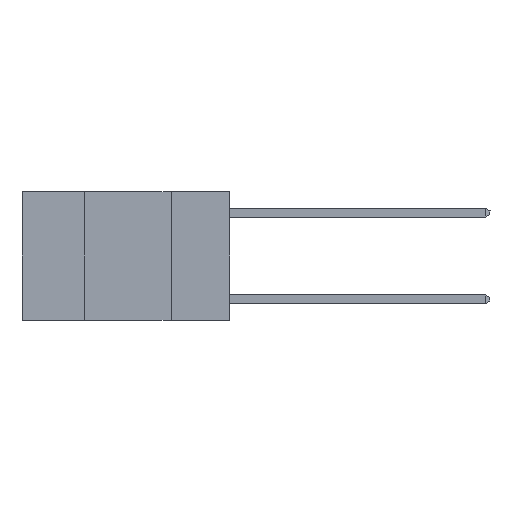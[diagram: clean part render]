
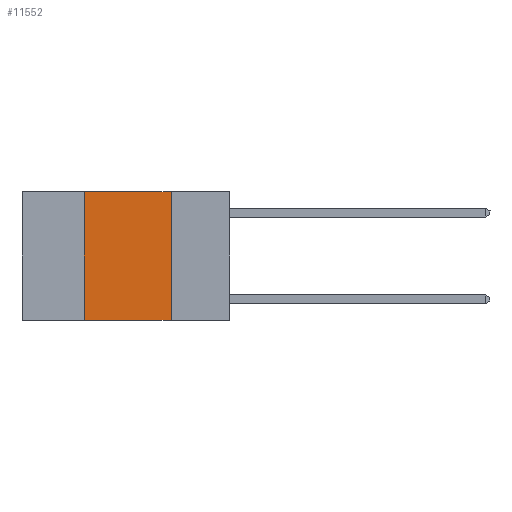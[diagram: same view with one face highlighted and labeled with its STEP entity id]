
A CAD part, left-side view. The second image highlights one B-rep face of the part: STEP entity #11552.
In plain terms, the highlighted planar face has unit normal (-1, 0, 0).
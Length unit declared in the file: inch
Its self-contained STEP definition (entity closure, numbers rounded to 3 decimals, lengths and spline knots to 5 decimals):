
#292 = LINE ( 'NONE', #2393, #14586 ) ;
#581 = CARTESIAN_POINT ( 'NONE',  ( 0., 0.17, -0.37 ) ) ;
#664 = EDGE_CURVE ( 'NONE', #5744, #1374, #12304, .T. ) ;
#1374 = VERTEX_POINT ( 'NONE', #581 ) ;
#2301 = VECTOR ( 'NONE', #14148, 39.37008 ) ;
#2393 = CARTESIAN_POINT ( 'NONE',  ( 0., 0.42, 0. ) ) ;
#2419 = EDGE_CURVE ( 'NONE', #4407, #1374, #6456, .T. ) ;
#2503 = EDGE_CURVE ( 'NONE', #4302, #5744, #11061, .T. ) ;
#3565 = DIRECTION ( 'NONE',  ( 0., 0., 1. ) ) ;
#4302 = VERTEX_POINT ( 'NONE', #5931 ) ;
#4407 = VERTEX_POINT ( 'NONE', #4926 ) ;
#4926 = CARTESIAN_POINT ( 'NONE',  ( 0., 0.42, -0.37 ) ) ;
#5465 = CARTESIAN_POINT ( 'NONE',  ( 0., 0.17, 0. ) ) ;
#5655 = DIRECTION ( 'NONE',  ( 1., 0., 0. ) ) ;
#5744 = VERTEX_POINT ( 'NONE', #7036 ) ;
#5931 = CARTESIAN_POINT ( 'NONE',  ( 0., 0.42, 0. ) ) ;
#6369 = CARTESIAN_POINT ( 'NONE',  ( 0., 0.6, 0. ) ) ;
#6412 = EDGE_CURVE ( 'NONE', #4407, #4302, #292, .T. ) ;
#6456 = LINE ( 'NONE', #13839, #9117 ) ;
#6716 = ORIENTED_EDGE ( 'NONE', *, *, #664, .F. ) ;
#7036 = CARTESIAN_POINT ( 'NONE',  ( 0., 0.17, 0. ) ) ;
#7872 = CARTESIAN_POINT ( 'NONE',  ( 0., 0.6, 0. ) ) ;
#9117 = VECTOR ( 'NONE', #12657, 39.37008 ) ;
#11061 = LINE ( 'NONE', #6369, #2301 ) ;
#11539 = AXIS2_PLACEMENT_3D ( 'NONE', #7872, #5655, #13462 ) ;
#11552 = ADVANCED_FACE ( 'NONE', ( #12076 ), #12385, .F. ) ;
#11667 = ORIENTED_EDGE ( 'NONE', *, *, #2503, .F. ) ;
#11950 = VECTOR ( 'NONE', #12206, 39.37008 ) ;
#12076 = FACE_OUTER_BOUND ( 'NONE', #14243, .T. ) ;
#12206 = DIRECTION ( 'NONE',  ( 0., 0., -1. ) ) ;
#12255 = ORIENTED_EDGE ( 'NONE', *, *, #6412, .F. ) ;
#12304 = LINE ( 'NONE', #5465, #11950 ) ;
#12385 = PLANE ( 'NONE',  #11539 ) ;
#12657 = DIRECTION ( 'NONE',  ( 0., -1., 0. ) ) ;
#12671 = ORIENTED_EDGE ( 'NONE', *, *, #2419, .T. ) ;
#13462 = DIRECTION ( 'NONE',  ( 0., 0., -1. ) ) ;
#13839 = CARTESIAN_POINT ( 'NONE',  ( 0., 0.6, -0.37 ) ) ;
#14148 = DIRECTION ( 'NONE',  ( 0., -1., 0. ) ) ;
#14243 = EDGE_LOOP ( 'NONE', ( #6716, #11667, #12255, #12671 ) ) ;
#14586 = VECTOR ( 'NONE', #3565, 39.37008 ) ;
